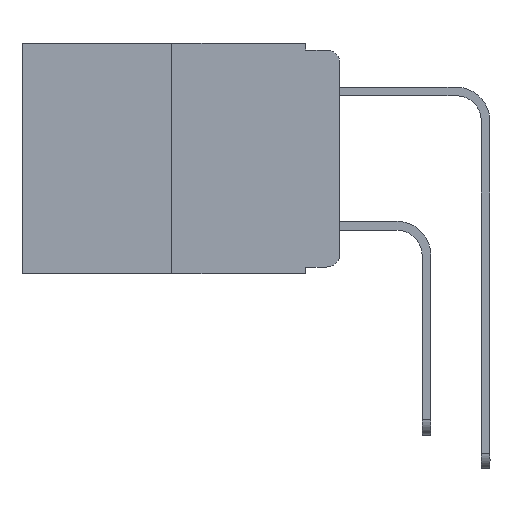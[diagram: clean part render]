
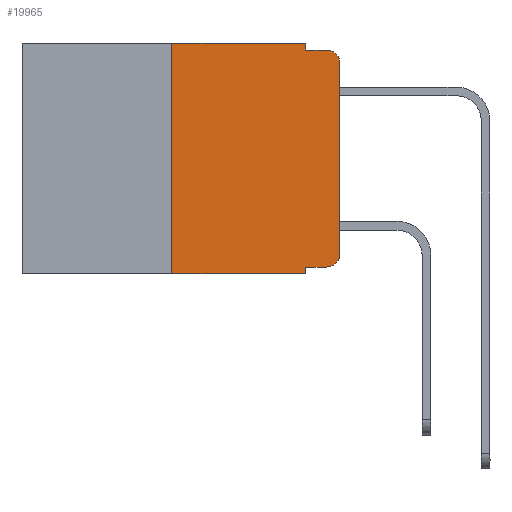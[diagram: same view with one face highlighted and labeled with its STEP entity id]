
A CAD part, left-side view. The second image highlights one B-rep face of the part: STEP entity #19965.
In plain terms, the highlighted planar face has unit normal (-1, 0, 0).
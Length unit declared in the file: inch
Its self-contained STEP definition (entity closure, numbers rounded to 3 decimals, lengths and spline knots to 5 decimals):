
#187 = CARTESIAN_POINT ( 'NONE',  ( 0., 0.051, 0. ) ) ;
#411 = DIRECTION ( 'NONE',  ( 0., 0., -1. ) ) ;
#790 = DIRECTION ( 'NONE',  ( -1., 0., 0. ) ) ;
#876 = VECTOR ( 'NONE', #13040, 39.37008 ) ;
#1517 = CARTESIAN_POINT ( 'NONE',  ( 0., 0.051, 0. ) ) ;
#1685 = CIRCLE ( 'NONE', #23262, 0.02 ) ;
#2369 = CARTESIAN_POINT ( 'NONE',  ( 0., 0.02, -0.333 ) ) ;
#2997 = ORIENTED_EDGE ( 'NONE', *, *, #14391, .F. ) ;
#3605 = PLANE ( 'NONE',  #24154 ) ;
#4221 = CARTESIAN_POINT ( 'NONE',  ( 0., 0.473, 0. ) ) ;
#4476 = ORIENTED_EDGE ( 'NONE', *, *, #14848, .T. ) ;
#4532 = AXIS2_PLACEMENT_3D ( 'NONE', #23136, #7772, #411 ) ;
#4581 = CARTESIAN_POINT ( 'NONE',  ( 0., 0.25, 0. ) ) ;
#4778 = ORIENTED_EDGE ( 'NONE', *, *, #9029, .F. ) ;
#5351 = CARTESIAN_POINT ( 'NONE',  ( 0., 0.25, -0.343 ) ) ;
#5406 = DIRECTION ( 'NONE',  ( 0., 0., 1. ) ) ;
#5457 = VECTOR ( 'NONE', #11280, 39.37008 ) ;
#6148 = EDGE_CURVE ( 'NONE', #18363, #15477, #10951, .T. ) ;
#6301 = DIRECTION ( 'NONE',  ( 0., -1., 0. ) ) ;
#6482 = VECTOR ( 'NONE', #9916, 39.37008 ) ;
#6927 = VERTEX_POINT ( 'NONE', #5351 ) ;
#7021 = LINE ( 'NONE', #1517, #14433 ) ;
#7074 = EDGE_CURVE ( 'NONE', #19710, #15477, #1685, .T. ) ;
#7473 = CARTESIAN_POINT ( 'NONE',  ( 0., 0.051, -0.333 ) ) ;
#7498 = CARTESIAN_POINT ( 'NONE',  ( 0., 0.051, -0.333 ) ) ;
#7628 = VERTEX_POINT ( 'NONE', #2369 ) ;
#7711 = VERTEX_POINT ( 'NONE', #21635 ) ;
#7772 = DIRECTION ( 'NONE',  ( -1., 0., 0. ) ) ;
#8194 = VECTOR ( 'NONE', #5406, 39.37008 ) ;
#8256 = DIRECTION ( 'NONE',  ( 0., 0., -1. ) ) ;
#8973 = CARTESIAN_POINT ( 'NONE',  ( 0., 0.25, 0. ) ) ;
#9029 = EDGE_CURVE ( 'NONE', #7711, #18363, #20547, .T. ) ;
#9220 = ORIENTED_EDGE ( 'NONE', *, *, #19995, .T. ) ;
#9305 = VECTOR ( 'NONE', #6301, 39.37008 ) ;
#9719 = EDGE_CURVE ( 'NONE', #22010, #19710, #21599, .T. ) ;
#9732 = DIRECTION ( 'NONE',  ( 1., 0., 0. ) ) ;
#9916 = DIRECTION ( 'NONE',  ( 0., 0., 1. ) ) ;
#10817 = CIRCLE ( 'NONE', #4532, 0.02 ) ;
#10838 = VERTEX_POINT ( 'NONE', #7498 ) ;
#10910 = ORIENTED_EDGE ( 'NONE', *, *, #11730, .F. ) ;
#10951 = LINE ( 'NONE', #22385, #876 ) ;
#11280 = DIRECTION ( 'NONE',  ( 0., -1., 0. ) ) ;
#11355 = ORIENTED_EDGE ( 'NONE', *, *, #21360, .T. ) ;
#11380 = VERTEX_POINT ( 'NONE', #14419 ) ;
#11730 = EDGE_CURVE ( 'NONE', #21262, #7711, #17223, .T. ) ;
#11783 = EDGE_LOOP ( 'NONE', ( #14192, #12662, #20840, #4778, #10910, #22162, #11355, #2997, #4476, #9220 ) ) ;
#11984 = CARTESIAN_POINT ( 'NONE',  ( 0., 0.02, -0.01 ) ) ;
#12068 = CARTESIAN_POINT ( 'NONE',  ( 0., 0.473, 0. ) ) ;
#12662 = ORIENTED_EDGE ( 'NONE', *, *, #7074, .T. ) ;
#12945 = FACE_OUTER_BOUND ( 'NONE', #11783, .T. ) ;
#13040 = DIRECTION ( 'NONE',  ( 0., -1., 0. ) ) ;
#13129 = LINE ( 'NONE', #7473, #5457 ) ;
#13538 = DIRECTION ( 'NONE',  ( 0., -1., 0. ) ) ;
#13588 = VECTOR ( 'NONE', #13538, 39.37008 ) ;
#13670 = CARTESIAN_POINT ( 'NONE',  ( 0., 0.02, -0.03 ) ) ;
#14192 = ORIENTED_EDGE ( 'NONE', *, *, #9719, .T. ) ;
#14391 = EDGE_CURVE ( 'NONE', #10838, #11380, #7021, .T. ) ;
#14419 = CARTESIAN_POINT ( 'NONE',  ( 0., 0.051, -0.343 ) ) ;
#14433 = VECTOR ( 'NONE', #18657, 39.37008 ) ;
#14741 = EDGE_CURVE ( 'NONE', #6927, #21262, #16448, .T. ) ;
#14848 = EDGE_CURVE ( 'NONE', #10838, #7628, #13129, .T. ) ;
#15419 = CARTESIAN_POINT ( 'NONE',  ( 0., 0., 0. ) ) ;
#15477 = VERTEX_POINT ( 'NONE', #11984 ) ;
#16209 = CARTESIAN_POINT ( 'NONE',  ( 0., 0., -0.313 ) ) ;
#16448 = LINE ( 'NONE', #8973, #8194 ) ;
#17223 = LINE ( 'NONE', #4221, #9305 ) ;
#17336 = LINE ( 'NONE', #22892, #13588 ) ;
#18363 = VERTEX_POINT ( 'NONE', #19437 ) ;
#18657 = DIRECTION ( 'NONE',  ( 0., 0., -1. ) ) ;
#19437 = CARTESIAN_POINT ( 'NONE',  ( 0., 0.051, -0.01 ) ) ;
#19710 = VERTEX_POINT ( 'NONE', #23531 ) ;
#19965 = ADVANCED_FACE ( 'NONE', ( #12945 ), #3605, .F. ) ;
#19995 = EDGE_CURVE ( 'NONE', #7628, #22010, #10817, .T. ) ;
#20547 = LINE ( 'NONE', #187, #23726 ) ;
#20840 = ORIENTED_EDGE ( 'NONE', *, *, #6148, .F. ) ;
#21262 = VERTEX_POINT ( 'NONE', #4581 ) ;
#21289 = DIRECTION ( 'NONE',  ( 0., 0., -1. ) ) ;
#21360 = EDGE_CURVE ( 'NONE', #6927, #11380, #17336, .T. ) ;
#21391 = DIRECTION ( 'NONE',  ( 0., 0., -1. ) ) ;
#21599 = LINE ( 'NONE', #15419, #6482 ) ;
#21635 = CARTESIAN_POINT ( 'NONE',  ( 0., 0.051, 0. ) ) ;
#22010 = VERTEX_POINT ( 'NONE', #16209 ) ;
#22162 = ORIENTED_EDGE ( 'NONE', *, *, #14741, .F. ) ;
#22385 = CARTESIAN_POINT ( 'NONE',  ( 0., 0.051, -0.01 ) ) ;
#22892 = CARTESIAN_POINT ( 'NONE',  ( 0., 0.473, -0.343 ) ) ;
#23136 = CARTESIAN_POINT ( 'NONE',  ( 0., 0.02, -0.313 ) ) ;
#23262 = AXIS2_PLACEMENT_3D ( 'NONE', #13670, #790, #21289 ) ;
#23531 = CARTESIAN_POINT ( 'NONE',  ( 0., 0., -0.03 ) ) ;
#23726 = VECTOR ( 'NONE', #21391, 39.37008 ) ;
#24154 = AXIS2_PLACEMENT_3D ( 'NONE', #12068, #9732, #8256 ) ;
